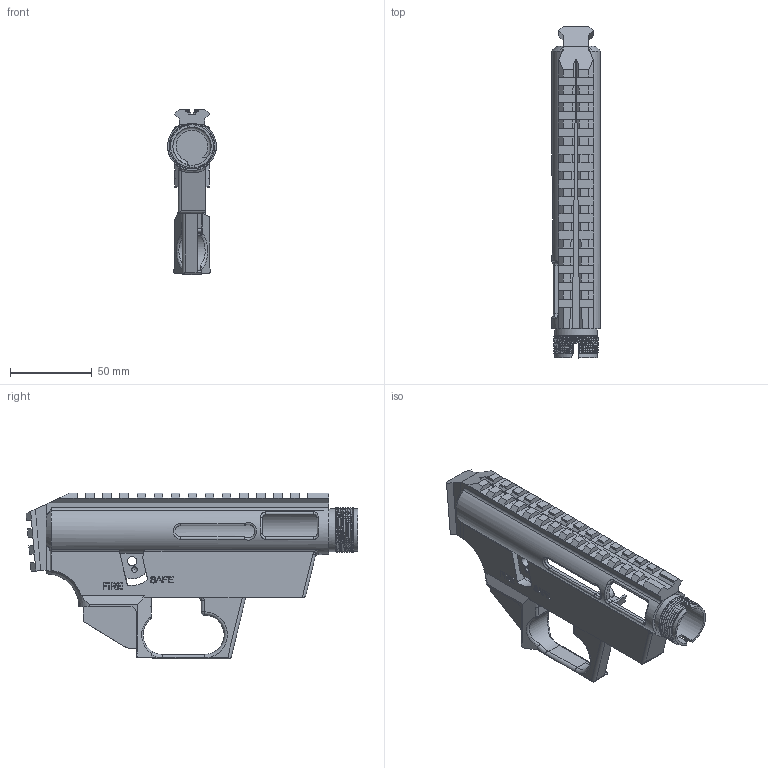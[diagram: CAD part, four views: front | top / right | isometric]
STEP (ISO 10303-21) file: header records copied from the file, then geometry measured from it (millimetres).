
FILE_DESCRIPTION(/* description */ (''),/* implementation_level */ '2;1');
FILE_NAME(/* name */ 'AR-7 Camper III v8.step',/* time_stamp */ '2020-12-07T22:03:40-05:00',/* author */ (''),/* organization */ (''),/* preprocessor_version */ 'ST-DEVELOPER v18.1',/* originating_system */ 'Autodesk Translation Framework v9.3.0.1241',/* authorisation */ '');
FILE_SCHEMA (('AUTOMOTIVE_DESIGN { 1 0 10303 214 3 1 1 }'));
Length unit declared in the file: millimetre
Products named in the file (2): AR-7 Camper III; Pistol Grip Assembly
Assembly tree (1 placements, depth 2):
  AR-7 Camper III
    Pistol Grip Assembly
Bounding box: 29.85 x 203.29 x 101.34 mm (x, y, z)
Volume: 130597.4 mm3; surface area: 55030.5 mm2
Topology: 2 solids, 2 shells, 685 faces, 1908 edges, 1237 vertices
Faces by surface type: plane 441, cylinder 120, bspline 100, torus 11, cone 9, sphere 4
Full cylindrical faces by diameter (mm): 3.45 x1, 3.75 x2, 3.95 x1, 4.3 x1, 5.65 x1, 7 x1, 7.75 x1, 23.4 x1, 26.132 x2, 26.3 x1, 27.85 x3
Entity records: 25696 total; most frequent: CARTESIAN_POINT 8745, ORIENTED_EDGE 3812, DIRECTION 3062, EDGE_CURVE 1906, LINE 1356, VECTOR 1356, VERTEX_POINT 1237, AXIS2_PLACEMENT_3D 853
